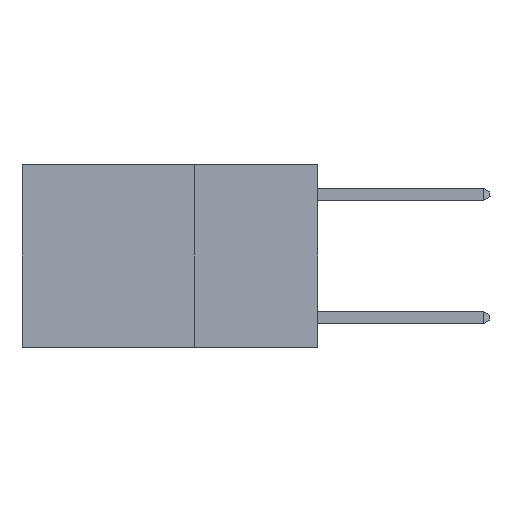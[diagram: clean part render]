
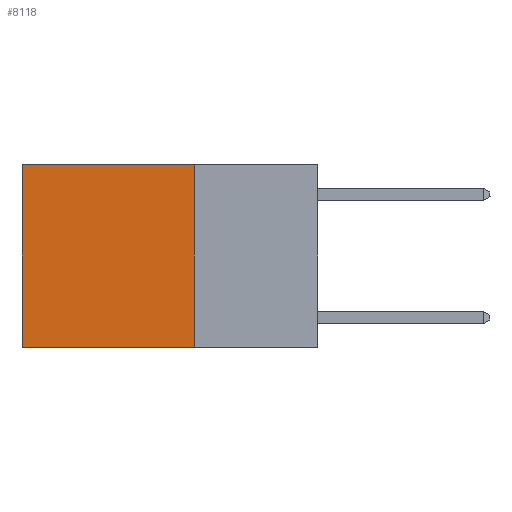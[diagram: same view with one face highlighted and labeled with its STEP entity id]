
A CAD part, left-side view. The second image highlights one B-rep face of the part: STEP entity #8118.
In plain terms, the highlighted planar face has unit normal (-1, 0, 0).
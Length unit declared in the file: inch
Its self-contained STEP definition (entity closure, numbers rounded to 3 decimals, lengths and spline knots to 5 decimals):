
#62 = PLANE ( 'NONE',  #5341 ) ;
#129 = LINE ( 'NONE', #971, #259 ) ;
#177 = CARTESIAN_POINT ( 'NONE',  ( 0.2625, 0.6, 0. ) ) ;
#259 = VECTOR ( 'NONE', #9405, 39.37008 ) ;
#971 = CARTESIAN_POINT ( 'NONE',  ( 0.2625, 0.6, 0. ) ) ;
#980 = VECTOR ( 'NONE', #3951, 39.37008 ) ;
#1197 = VERTEX_POINT ( 'NONE', #177 ) ;
#2085 = DIRECTION ( 'NONE',  ( 0., 1., 0. ) ) ;
#2481 = DIRECTION ( 'NONE',  ( 0., 0., -1. ) ) ;
#2533 = FACE_OUTER_BOUND ( 'NONE', #5748, .T. ) ;
#2560 = VECTOR ( 'NONE', #2085, 39.37008 ) ;
#2650 = DIRECTION ( 'NONE',  ( 1., 0., 0. ) ) ;
#2830 = CARTESIAN_POINT ( 'NONE',  ( 0.2625, 0.25, 0. ) ) ;
#3951 = DIRECTION ( 'NONE',  ( 0., 0., -1. ) ) ;
#3993 = ORIENTED_EDGE ( 'NONE', *, *, #9887, .F. ) ;
#4024 = EDGE_CURVE ( 'NONE', #9183, #1197, #6937, .T. ) ;
#4140 = CARTESIAN_POINT ( 'NONE',  ( 0.2625, 0.25, -0.37 ) ) ;
#4781 = LINE ( 'NONE', #5796, #980 ) ;
#5341 = AXIS2_PLACEMENT_3D ( 'NONE', #5927, #2650, #2481 ) ;
#5723 = CARTESIAN_POINT ( 'NONE',  ( 0.2625, 0.6, -0.37 ) ) ;
#5748 = EDGE_LOOP ( 'NONE', ( #8716, #3993, #8063, #6147 ) ) ;
#5796 = CARTESIAN_POINT ( 'NONE',  ( 0.2625, 0.25, 0. ) ) ;
#5927 = CARTESIAN_POINT ( 'NONE',  ( 0.2625, 0.25, 0. ) ) ;
#6009 = VERTEX_POINT ( 'NONE', #6030 ) ;
#6030 = CARTESIAN_POINT ( 'NONE',  ( 0.2625, 0.25, -0.37 ) ) ;
#6147 = ORIENTED_EDGE ( 'NONE', *, *, #4024, .T. ) ;
#6937 = LINE ( 'NONE', #10410, #2560 ) ;
#7148 = EDGE_CURVE ( 'NONE', #9183, #6009, #4781, .T. ) ;
#7757 = DIRECTION ( 'NONE',  ( 0., 1., 0. ) ) ;
#8063 = ORIENTED_EDGE ( 'NONE', *, *, #7148, .F. ) ;
#8118 = ADVANCED_FACE ( 'NONE', ( #2533 ), #62, .F. ) ;
#8716 = ORIENTED_EDGE ( 'NONE', *, *, #9346, .T. ) ;
#8891 = VERTEX_POINT ( 'NONE', #5723 ) ;
#9183 = VERTEX_POINT ( 'NONE', #2830 ) ;
#9275 = LINE ( 'NONE', #4140, #10247 ) ;
#9346 = EDGE_CURVE ( 'NONE', #1197, #8891, #129, .T. ) ;
#9405 = DIRECTION ( 'NONE',  ( 0., 0., -1. ) ) ;
#9887 = EDGE_CURVE ( 'NONE', #6009, #8891, #9275, .T. ) ;
#10247 = VECTOR ( 'NONE', #7757, 39.37008 ) ;
#10410 = CARTESIAN_POINT ( 'NONE',  ( 0.2625, 0.25, 0. ) ) ;
